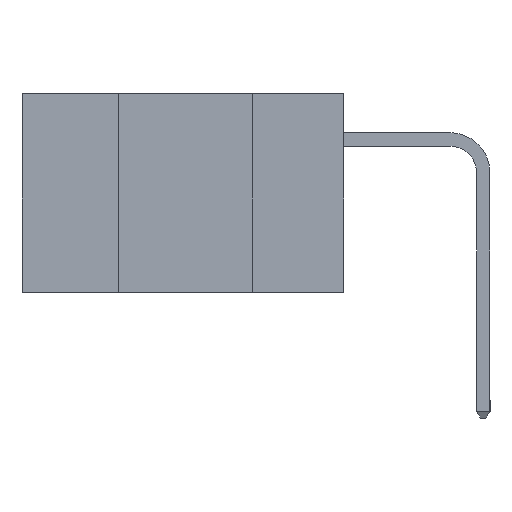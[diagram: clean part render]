
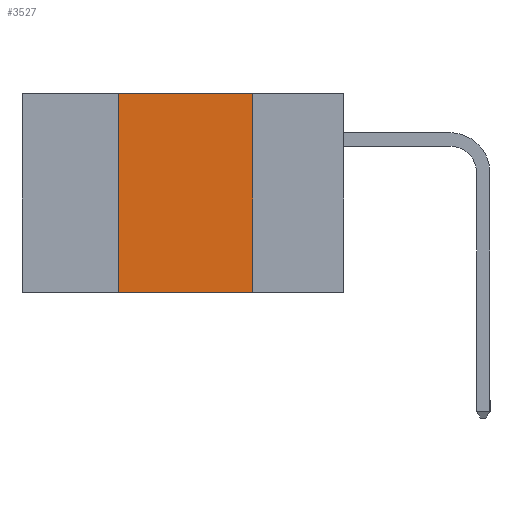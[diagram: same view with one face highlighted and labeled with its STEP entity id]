
A CAD part, left-side view. The second image highlights one B-rep face of the part: STEP entity #3527.
In plain terms, the highlighted planar face has unit normal (-1, 0, 0).
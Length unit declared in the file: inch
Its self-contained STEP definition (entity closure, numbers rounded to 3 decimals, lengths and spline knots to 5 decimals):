
#739 = AXIS2_PLACEMENT_3D ( 'NONE', #3343, #3293, #3204 ) ;
#1810 = DIRECTION ( 'NONE',  ( 0., 0., -1. ) ) ;
#1833 = EDGE_CURVE ( 'NONE', #15585, #7613, #7619, .T. ) ;
#1889 = ORIENTED_EDGE ( 'NONE', *, *, #13753, .F. ) ;
#2681 = LINE ( 'NONE', #6959, #5712 ) ;
#3116 = ORIENTED_EDGE ( 'NONE', *, *, #16460, .T. ) ;
#3204 = DIRECTION ( 'NONE',  ( 0., 0., -1. ) ) ;
#3293 = DIRECTION ( 'NONE',  ( 1., 0., 0. ) ) ;
#3343 = CARTESIAN_POINT ( 'NONE',  ( 0., 0.6, 0. ) ) ;
#3448 = PLANE ( 'NONE',  #739 ) ;
#3527 = ADVANCED_FACE ( 'NONE', ( #3915 ), #3448, .F. ) ;
#3915 = FACE_OUTER_BOUND ( 'NONE', #16228, .T. ) ;
#4622 = VECTOR ( 'NONE', #16291, 39.37008 ) ;
#5009 = VECTOR ( 'NONE', #15198, 39.37008 ) ;
#5062 = CARTESIAN_POINT ( 'NONE',  ( 0., 0.6, -0.37 ) ) ;
#5712 = VECTOR ( 'NONE', #1810, 39.37008 ) ;
#5726 = VERTEX_POINT ( 'NONE', #14267 ) ;
#5755 = CARTESIAN_POINT ( 'NONE',  ( 0., 0.6, 0. ) ) ;
#6477 = CARTESIAN_POINT ( 'NONE',  ( 0., 0.17, 0. ) ) ;
#6959 = CARTESIAN_POINT ( 'NONE',  ( 0., 0.17, -0.37 ) ) ;
#7478 = CARTESIAN_POINT ( 'NONE',  ( 0., 0.17, -0.37 ) ) ;
#7613 = VERTEX_POINT ( 'NONE', #6477 ) ;
#7619 = LINE ( 'NONE', #5755, #11404 ) ;
#10071 = ORIENTED_EDGE ( 'NONE', *, *, #12620, .F. ) ;
#11404 = VECTOR ( 'NONE', #16477, 39.37008 ) ;
#11704 = VERTEX_POINT ( 'NONE', #7478 ) ;
#12620 = EDGE_CURVE ( 'NONE', #7613, #11704, #2681, .T. ) ;
#13618 = CARTESIAN_POINT ( 'NONE',  ( 0., 0.42, 0. ) ) ;
#13753 = EDGE_CURVE ( 'NONE', #5726, #15585, #14686, .T. ) ;
#14161 = ORIENTED_EDGE ( 'NONE', *, *, #1833, .F. ) ;
#14267 = CARTESIAN_POINT ( 'NONE',  ( 0., 0.42, -0.37 ) ) ;
#14686 = LINE ( 'NONE', #15052, #4622 ) ;
#15052 = CARTESIAN_POINT ( 'NONE',  ( 0., 0.42, -0.37 ) ) ;
#15057 = LINE ( 'NONE', #5062, #5009 ) ;
#15198 = DIRECTION ( 'NONE',  ( 0., -1., 0. ) ) ;
#15585 = VERTEX_POINT ( 'NONE', #13618 ) ;
#16228 = EDGE_LOOP ( 'NONE', ( #10071, #14161, #1889, #3116 ) ) ;
#16291 = DIRECTION ( 'NONE',  ( 0., 0., 1. ) ) ;
#16460 = EDGE_CURVE ( 'NONE', #5726, #11704, #15057, .T. ) ;
#16477 = DIRECTION ( 'NONE',  ( 0., -1., 0. ) ) ;
